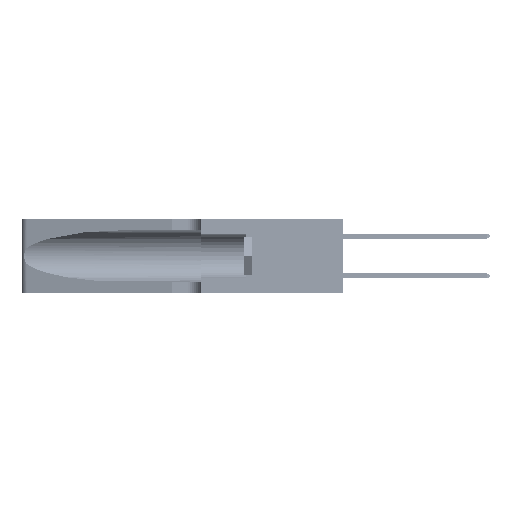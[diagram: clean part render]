
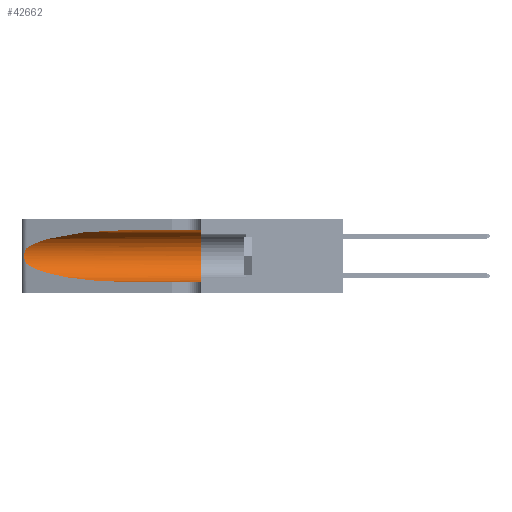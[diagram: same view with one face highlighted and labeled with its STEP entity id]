
A CAD part, left-side view. The second image highlights one B-rep face of the part: STEP entity #42662.
In plain terms, the highlighted cylindrical face has radius 3.308 mm (diameter 6.617 mm), a partial arc.
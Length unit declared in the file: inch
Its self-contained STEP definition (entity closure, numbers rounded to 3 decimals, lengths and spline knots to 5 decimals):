
#28 = CARTESIAN_POINT ( 'NONE',  ( 0.1305, 0.35, 0.05475 ) ) ;
#1128 = CARTESIAN_POINT ( 'NONE',  ( 0.1305, 0.35, 0.185 ) ) ;
#3045 = DIRECTION ( 'NONE',  ( 0., -1., 0. ) ) ;
#5043 = CARTESIAN_POINT ( 'NONE',  ( 0.25487, 1.22718, 0.14631 ) ) ;
#5155 = DIRECTION ( 'NONE',  ( 0., 1., 0. ) ) ;
#5715 = ORIENTED_EDGE ( 'NONE', *, *, #40359, .F. ) ;
#6727 = VECTOR ( 'NONE', #49405, 39.37008 ) ;
#6754 = CARTESIAN_POINT ( 'NONE',  ( 0.18966, 0.96281, 0.31525 ) ) ;
#7108 = DIRECTION ( 'NONE',  ( 0., 0., -1. ) ) ;
#7408 = CARTESIAN_POINT ( 'NONE',  ( 0.2373, 1.15595, 0.08982 ) ) ;
#9884 = EDGE_CURVE ( 'NONE', #27476, #35733, #33881, .T. ) ;
#11217 = VERTEX_POINT ( 'NONE', #37954 ) ;
#11978 = CARTESIAN_POINT ( 'NONE',  ( 0.25487, 1.22718, 0.14631 ) ) ;
#15390 = EDGE_CURVE ( 'NONE', #11217, #25004, #40962, .T. ) ;
#15458 = CARTESIAN_POINT ( 'NONE',  ( 0.25856, 1.23593, 0.16098 ) ) ;
#15805 = VERTEX_POINT ( 'NONE', #29200 ) ;
#15920 = CYLINDRICAL_SURFACE ( 'NONE', #47311, 0.13025 ) ;
#19400 = LINE ( 'NONE', #34220, #47709 ) ;
#19506 = CARTESIAN_POINT ( 'NONE',  ( 0.25854, 1.2359, 0.20912 ) ) ;
#19854 = CARTESIAN_POINT ( 'NONE',  ( 0.25787, 1.23484, 0.2124 ) ) ;
#20000 = VERTEX_POINT ( 'NONE', #44031 ) ;
#20973 = AXIS2_PLACEMENT_3D ( 'NONE', #1128, #5155, #33206 ) ;
#21305 = B_SPLINE_CURVE_WITH_KNOTS ( 'NONE', 3,
 ( #27747, #23338, #28095, #19854, #19506, #35486, #47987, #27923, #31446, #15458, #31975, #47632, #24035, #11978 ),
 .UNSPECIFIED., .F., .F.,
 ( 4, 2, 2, 2, 2, 2, 4 ),
 ( 0., 0.00027, 0.00053, 0.00107, 0.0016, 0.00187, 0.00214 ),
 .UNSPECIFIED. ) ;
#23175 = CARTESIAN_POINT ( 'NONE',  ( 0.1305, 1.61858, 0.185 ) ) ;
#23338 = CARTESIAN_POINT ( 'NONE',  ( 0.25555, 1.22994, 0.2215 ) ) ;
#23623 = LINE ( 'NONE', #29323, #6727 ) ;
#24035 = CARTESIAN_POINT ( 'NONE',  ( 0.25555, 1.22993, 0.14849 ) ) ;
#24261 = EDGE_LOOP ( 'NONE', ( #40288, #26913, #29275, #43524, #25357, #5715 ) ) ;
#24312 = CARTESIAN_POINT ( 'NONE',  ( 0.1305, 0.72297, 0.05475 ) ) ;
#25004 = VERTEX_POINT ( 'NONE', #28 ) ;
#25357 = ORIENTED_EDGE ( 'NONE', *, *, #15390, .F. ) ;
#26913 = ORIENTED_EDGE ( 'NONE', *, *, #40048, .T. ) ;
#27476 = VERTEX_POINT ( 'NONE', #5043 ) ;
#27747 = CARTESIAN_POINT ( 'NONE',  ( 0.25487, 1.22718, 0.22369 ) ) ;
#27863 = FACE_OUTER_BOUND ( 'NONE', #24261, .T. ) ;
#27923 = CARTESIAN_POINT ( 'NONE',  ( 0.26075, 1.23896, 0.178 ) ) ;
#28095 = CARTESIAN_POINT ( 'NONE',  ( 0.25639, 1.23184, 0.21858 ) ) ;
#29200 = CARTESIAN_POINT ( 'NONE',  ( 0.1305, 0.72297, 0.31525 ) ) ;
#29275 = ORIENTED_EDGE ( 'NONE', *, *, #9884, .T. ) ;
#29323 = CARTESIAN_POINT ( 'NONE',  ( 0.1305, 1.61858, 0.05475 ) ) ;
#30505 = DIRECTION ( 'NONE',  ( 0., -1., 0. ) ) ;
#31254 = EDGE_CURVE ( 'NONE', #35733, #25004, #23623, .T. ) ;
#31446 = CARTESIAN_POINT ( 'NONE',  ( 0.26017, 1.23833, 0.17102 ) ) ;
#31944 = CARTESIAN_POINT ( 'NONE',  ( 0.25487, 1.22718, 0.14631 ) ) ;
#31975 = CARTESIAN_POINT ( 'NONE',  ( 0.25789, 1.23486, 0.15765 ) ) ;
#33206 = DIRECTION ( 'NONE',  ( 0., 0., 1. ) ) ;
#33266 = CARTESIAN_POINT ( 'NONE',  ( 0.2373, 1.15595, 0.28018 ) ) ;
#33881 =( BOUNDED_CURVE ( )  B_SPLINE_CURVE ( 3, ( #31944, #7408, #47607, #39628 ),
 .UNSPECIFIED., .F., .F. ) 
 B_SPLINE_CURVE_WITH_KNOTS ( ( 4, 4 ),
 ( 3.44316, 4.71239 ),
 .UNSPECIFIED. ) 
 CURVE ( )  GEOMETRIC_REPRESENTATION_ITEM ( )  RATIONAL_B_SPLINE_CURVE ( ( 1., 0.87, 0.87, 1. ) ) 
 REPRESENTATION_ITEM ( '' )  );
#34220 = CARTESIAN_POINT ( 'NONE',  ( 0.1305, 1.61858, 0.31525 ) ) ;
#35486 = CARTESIAN_POINT ( 'NONE',  ( 0.26018, 1.23835, 0.19895 ) ) ;
#35733 = VERTEX_POINT ( 'NONE', #24312 ) ;
#37954 = CARTESIAN_POINT ( 'NONE',  ( 0.1305, 0.35, 0.31525 ) ) ;
#39628 = CARTESIAN_POINT ( 'NONE',  ( 0.1305, 0.72297, 0.05475 ) ) ;
#40048 = EDGE_CURVE ( 'NONE', #20000, #27476, #21305, .T. ) ;
#40288 = ORIENTED_EDGE ( 'NONE', *, *, #50835, .T. ) ;
#40359 = EDGE_CURVE ( 'NONE', #15805, #11217, #19400, .T. ) ;
#40962 = CIRCLE ( 'NONE', #20973, 0.13025 ) ;
#42122 = CARTESIAN_POINT ( 'NONE',  ( 0.1305, 0.72297, 0.31525 ) ) ;
#42662 = ADVANCED_FACE ( 'NONE', ( #27863 ), #15920, .F. ) ;
#43524 = ORIENTED_EDGE ( 'NONE', *, *, #31254, .T. ) ;
#44031 = CARTESIAN_POINT ( 'NONE',  ( 0.25487, 1.22718, 0.22369 ) ) ;
#45838 = CARTESIAN_POINT ( 'NONE',  ( 0.25487, 1.22718, 0.22369 ) ) ;
#47311 = AXIS2_PLACEMENT_3D ( 'NONE', #23175, #3045, #7108 ) ;
#47607 = CARTESIAN_POINT ( 'NONE',  ( 0.18966, 0.96281, 0.05475 ) ) ;
#47632 = CARTESIAN_POINT ( 'NONE',  ( 0.25639, 1.23186, 0.15144 ) ) ;
#47709 = VECTOR ( 'NONE', #30505, 39.37008 ) ;
#47987 = CARTESIAN_POINT ( 'NONE',  ( 0.26075, 1.23896, 0.19203 ) ) ;
#49405 = DIRECTION ( 'NONE',  ( 0., -1., 0. ) ) ;
#50336 =( BOUNDED_CURVE ( )  B_SPLINE_CURVE ( 3, ( #42122, #6754, #33266, #45838 ),
 .UNSPECIFIED., .F., .F. ) 
 B_SPLINE_CURVE_WITH_KNOTS ( ( 4, 4 ),
 ( 1.5708, 2.84003 ),
 .UNSPECIFIED. ) 
 CURVE ( )  GEOMETRIC_REPRESENTATION_ITEM ( )  RATIONAL_B_SPLINE_CURVE ( ( 1., 0.87, 0.87, 1. ) ) 
 REPRESENTATION_ITEM ( '' )  );
#50835 = EDGE_CURVE ( 'NONE', #15805, #20000, #50336, .T. ) ;
